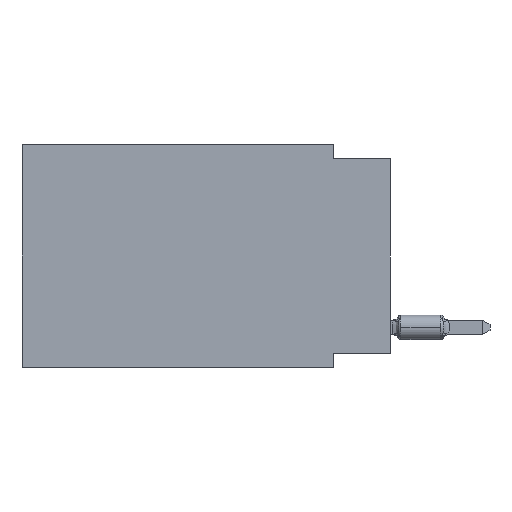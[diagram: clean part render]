
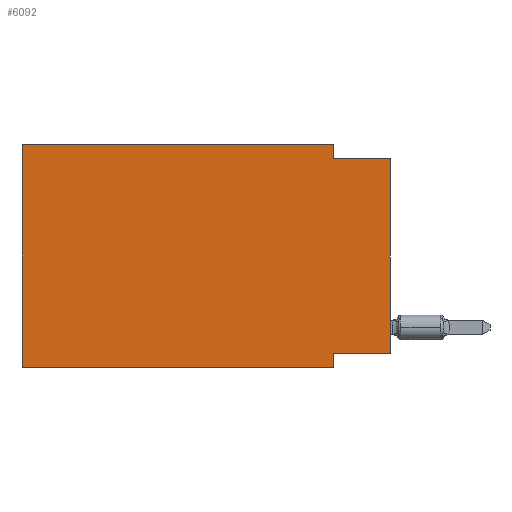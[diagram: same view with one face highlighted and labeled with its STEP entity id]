
A CAD part, left-side view. The second image highlights one B-rep face of the part: STEP entity #6092.
In plain terms, the highlighted planar face has unit normal (-1, 0, 0).
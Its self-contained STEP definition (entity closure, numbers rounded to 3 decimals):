
#531 = ORIENTED_EDGE ( 'NONE', *, *, #2617, .F. ) ;
#771 = ORIENTED_EDGE ( 'NONE', *, *, #12473, .F. ) ;
#1172 = DIRECTION ( 'NONE',  ( 1., 0., 0. ) ) ;
#1219 = CARTESIAN_POINT ( 'NONE',  ( 0., 16.383, -9.906 ) ) ;
#1455 = DIRECTION ( 'NONE',  ( 0., 0., 1. ) ) ;
#2076 = ORIENTED_EDGE ( 'NONE', *, *, #3904, .F. ) ;
#2617 = EDGE_CURVE ( 'NONE', #3402, #12924, #10023, .T. ) ;
#2644 = ORIENTED_EDGE ( 'NONE', *, *, #8751, .F. ) ;
#3035 = LINE ( 'NONE', #7489, #9070 ) ;
#3402 = VERTEX_POINT ( 'NONE', #8417 ) ;
#3444 = VERTEX_POINT ( 'NONE', #5545 ) ;
#3489 = VERTEX_POINT ( 'NONE', #10057 ) ;
#3494 = DIRECTION ( 'NONE',  ( 0., 0., -1. ) ) ;
#3543 = EDGE_CURVE ( 'NONE', #4104, #9834, #10195, .T. ) ;
#3803 = CARTESIAN_POINT ( 'NONE',  ( 0., 16.383, 0. ) ) ;
#3904 = EDGE_CURVE ( 'NONE', #9834, #3489, #5743, .T. ) ;
#4036 = DIRECTION ( 'NONE',  ( 0., 1., 0. ) ) ;
#4104 = VERTEX_POINT ( 'NONE', #12873 ) ;
#4206 = VECTOR ( 'NONE', #11386, 1000. ) ;
#4545 = DIRECTION ( 'NONE',  ( 0., -1., 0. ) ) ;
#4729 = CARTESIAN_POINT ( 'NONE',  ( 0., 0., 0. ) ) ;
#4767 = LINE ( 'NONE', #13442, #11890 ) ;
#4983 = CARTESIAN_POINT ( 'NONE',  ( 0., 16.383, 0. ) ) ;
#5394 = EDGE_CURVE ( 'NONE', #3489, #3402, #7949, .T. ) ;
#5539 = DIRECTION ( 'NONE',  ( 0., 0., -1. ) ) ;
#5545 = CARTESIAN_POINT ( 'NONE',  ( 0., 2.54, -9.271 ) ) ;
#5743 = LINE ( 'NONE', #6882, #4206 ) ;
#6092 = ADVANCED_FACE ( 'NONE', ( #10487 ), #9443, .F. ) ;
#6191 = EDGE_CURVE ( 'NONE', #8150, #12924, #7830, .T. ) ;
#6882 = CARTESIAN_POINT ( 'NONE',  ( 0., 16.383, 0. ) ) ;
#7489 = CARTESIAN_POINT ( 'NONE',  ( 0., 0., -9.271 ) ) ;
#7633 = VECTOR ( 'NONE', #11949, 1000. ) ;
#7830 = LINE ( 'NONE', #4729, #13476 ) ;
#7867 = ORIENTED_EDGE ( 'NONE', *, *, #5394, .F. ) ;
#7949 = LINE ( 'NONE', #13315, #12430 ) ;
#8041 = VECTOR ( 'NONE', #4545, 1000. ) ;
#8150 = VERTEX_POINT ( 'NONE', #10175 ) ;
#8268 = VECTOR ( 'NONE', #1455, 1000. ) ;
#8417 = CARTESIAN_POINT ( 'NONE',  ( 0., 2.54, -0.635 ) ) ;
#8453 = ORIENTED_EDGE ( 'NONE', *, *, #13664, .T. ) ;
#8751 = EDGE_CURVE ( 'NONE', #8150, #3444, #3035, .T. ) ;
#9070 = VECTOR ( 'NONE', #4036, 1000. ) ;
#9137 = DIRECTION ( 'NONE',  ( 0., 0., 1. ) ) ;
#9153 = VERTEX_POINT ( 'NONE', #13761 ) ;
#9443 = PLANE ( 'NONE',  #9855 ) ;
#9834 = VERTEX_POINT ( 'NONE', #4983 ) ;
#9855 = AXIS2_PLACEMENT_3D ( 'NONE', #12050, #1172, #5539 ) ;
#10023 = LINE ( 'NONE', #11216, #8041 ) ;
#10057 = CARTESIAN_POINT ( 'NONE',  ( 0., 2.54, 0. ) ) ;
#10175 = CARTESIAN_POINT ( 'NONE',  ( 0., 0., -9.271 ) ) ;
#10195 = LINE ( 'NONE', #3803, #8268 ) ;
#10197 = CARTESIAN_POINT ( 'NONE',  ( 0., 0., -0.635 ) ) ;
#10487 = FACE_OUTER_BOUND ( 'NONE', #13228, .T. ) ;
#11139 = ORIENTED_EDGE ( 'NONE', *, *, #3543, .F. ) ;
#11216 = CARTESIAN_POINT ( 'NONE',  ( 0., 0., -0.635 ) ) ;
#11369 = DIRECTION ( 'NONE',  ( 0., 0., -1. ) ) ;
#11386 = DIRECTION ( 'NONE',  ( 0., -1., 0. ) ) ;
#11890 = VECTOR ( 'NONE', #11369, 1000. ) ;
#11949 = DIRECTION ( 'NONE',  ( 0., -1., 0. ) ) ;
#12050 = CARTESIAN_POINT ( 'NONE',  ( 0., 16.383, 0. ) ) ;
#12430 = VECTOR ( 'NONE', #3494, 1000. ) ;
#12473 = EDGE_CURVE ( 'NONE', #3444, #9153, #4767, .T. ) ;
#12744 = ORIENTED_EDGE ( 'NONE', *, *, #6191, .T. ) ;
#12873 = CARTESIAN_POINT ( 'NONE',  ( 0., 16.383, -9.906 ) ) ;
#12924 = VERTEX_POINT ( 'NONE', #10197 ) ;
#13018 = LINE ( 'NONE', #1219, #7633 ) ;
#13228 = EDGE_LOOP ( 'NONE', ( #12744, #531, #7867, #2076, #11139, #8453, #771, #2644 ) ) ;
#13315 = CARTESIAN_POINT ( 'NONE',  ( 0., 2.54, 0. ) ) ;
#13442 = CARTESIAN_POINT ( 'NONE',  ( 0., 2.54, -9.906 ) ) ;
#13476 = VECTOR ( 'NONE', #9137, 1000. ) ;
#13664 = EDGE_CURVE ( 'NONE', #4104, #9153, #13018, .T. ) ;
#13761 = CARTESIAN_POINT ( 'NONE',  ( 0., 2.54, -9.906 ) ) ;
